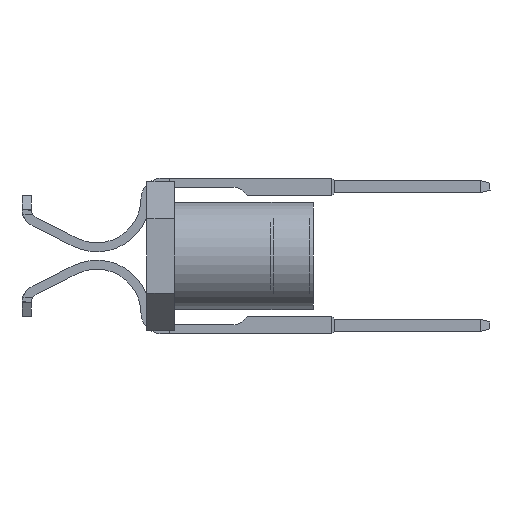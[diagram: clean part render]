
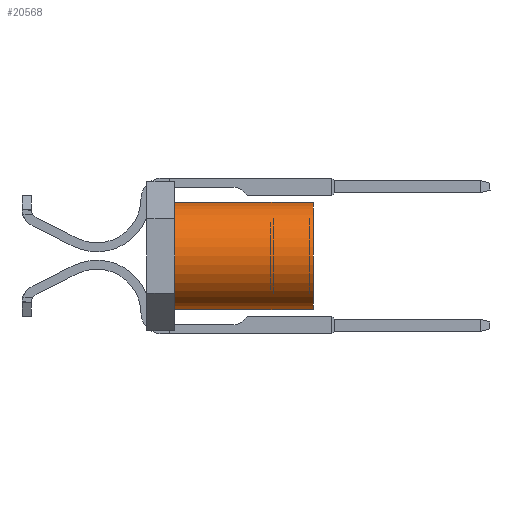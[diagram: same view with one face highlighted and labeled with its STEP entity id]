
A CAD part, left-side view. The second image highlights one B-rep face of the part: STEP entity #20568.
In plain terms, the highlighted cylindrical face has radius 1.968 mm (diameter 3.937 mm), a partial arc.
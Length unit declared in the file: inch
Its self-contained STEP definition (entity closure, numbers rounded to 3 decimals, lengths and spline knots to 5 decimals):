
#518 = ORIENTED_EDGE ( 'NONE', *, *, #8555, .T. ) ;
#1191 = VERTEX_POINT ( 'NONE', #19232 ) ;
#1990 = CARTESIAN_POINT ( 'NONE',  ( 0., 0.24, 0. ) ) ;
#2550 = DIRECTION ( 'NONE',  ( 0., 0., 1. ) ) ;
#8555 = EDGE_CURVE ( 'NONE', #17750, #14894, #14224, .T. ) ;
#9268 = CIRCLE ( 'NONE', #33171, 0.0775 ) ;
#9566 = DIRECTION ( 'NONE',  ( 0., 0., 1. ) ) ;
#11225 = CARTESIAN_POINT ( 'NONE',  ( 0., 0.04, 0.0775 ) ) ;
#13591 = ORIENTED_EDGE ( 'NONE', *, *, #40082, .F. ) ;
#14224 = LINE ( 'NONE', #27274, #14729 ) ;
#14729 = VECTOR ( 'NONE', #39675, 39.37008 ) ;
#14894 = VERTEX_POINT ( 'NONE', #33660 ) ;
#17261 = AXIS2_PLACEMENT_3D ( 'NONE', #29026, #38835, #9566 ) ;
#17750 = VERTEX_POINT ( 'NONE', #27586 ) ;
#19232 = CARTESIAN_POINT ( 'NONE',  ( 0., 0.24, 0.0775 ) ) ;
#19619 = DIRECTION ( 'NONE',  ( 0., 1., 0. ) ) ;
#20568 = ADVANCED_FACE ( 'NONE', ( #31474 ), #28048, .T. ) ;
#21433 = CARTESIAN_POINT ( 'NONE',  ( 0., 0.24, 0.0775 ) ) ;
#21649 = DIRECTION ( 'NONE',  ( 0., 0., -1. ) ) ;
#23042 = CARTESIAN_POINT ( 'NONE',  ( 0., 0.24, 0. ) ) ;
#24855 = DIRECTION ( 'NONE',  ( 0., -1., 0. ) ) ;
#25048 = LINE ( 'NONE', #21433, #39836 ) ;
#27091 = AXIS2_PLACEMENT_3D ( 'NONE', #1990, #24855, #21649 ) ;
#27274 = CARTESIAN_POINT ( 'NONE',  ( 0., 0.24, -0.0775 ) ) ;
#27406 = CIRCLE ( 'NONE', #17261, 0.0775 ) ;
#27586 = CARTESIAN_POINT ( 'NONE',  ( 0., 0.24, -0.0775 ) ) ;
#28048 = CYLINDRICAL_SURFACE ( 'NONE', #27091, 0.0775 ) ;
#29026 = CARTESIAN_POINT ( 'NONE',  ( 0., 0.04, 0. ) ) ;
#29949 = EDGE_LOOP ( 'NONE', ( #37239, #13591, #518, #34249 ) ) ;
#30435 = EDGE_CURVE ( 'NONE', #1191, #33056, #25048, .T. ) ;
#31474 = FACE_OUTER_BOUND ( 'NONE', #29949, .T. ) ;
#33056 = VERTEX_POINT ( 'NONE', #11225 ) ;
#33171 = AXIS2_PLACEMENT_3D ( 'NONE', #23042, #19619, #2550 ) ;
#33660 = CARTESIAN_POINT ( 'NONE',  ( 0., 0.04, -0.0775 ) ) ;
#34249 = ORIENTED_EDGE ( 'NONE', *, *, #34416, .T. ) ;
#34416 = EDGE_CURVE ( 'NONE', #14894, #33056, #27406, .T. ) ;
#37239 = ORIENTED_EDGE ( 'NONE', *, *, #30435, .F. ) ;
#37642 = DIRECTION ( 'NONE',  ( 0., -1., 0. ) ) ;
#38835 = DIRECTION ( 'NONE',  ( 0., 1., 0. ) ) ;
#39675 = DIRECTION ( 'NONE',  ( 0., -1., 0. ) ) ;
#39836 = VECTOR ( 'NONE', #37642, 39.37008 ) ;
#40082 = EDGE_CURVE ( 'NONE', #17750, #1191, #9268, .T. ) ;
